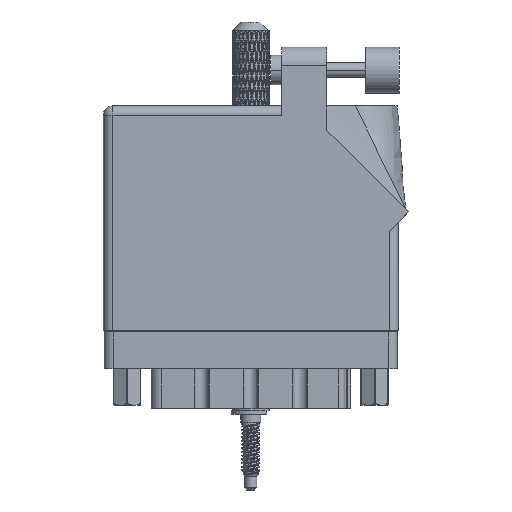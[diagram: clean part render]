
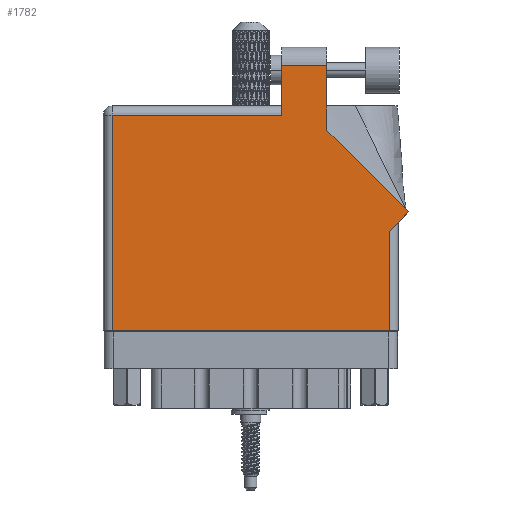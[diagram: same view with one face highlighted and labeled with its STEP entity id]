
A CAD part, front view. The second image highlights one B-rep face of the part: STEP entity #1782.
In plain terms, the highlighted face is planar.
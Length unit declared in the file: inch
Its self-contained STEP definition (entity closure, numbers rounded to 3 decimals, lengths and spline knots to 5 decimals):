
#1079 = CARTESIAN_POINT ( 'NONE',  ( 1.217, 1.468, 0. ) ) ;
#1595 = VERTEX_POINT ( 'NONE', #8621 ) ;
#1782 = ADVANCED_FACE ( 'NONE', ( #30222 ), #41674, .F. ) ;
#3000 = CARTESIAN_POINT ( 'NONE',  ( 1.524, 1.36442, 0. ) ) ;
#3484 = CARTESIAN_POINT ( 'NONE',  ( 0.062, 1.468, 0. ) ) ;
#4439 = DIRECTION ( 'NONE',  ( 0.707, 0.707, 0. ) ) ;
#5820 = DIRECTION ( 'NONE',  ( 0., 0., -1. ) ) ;
#7330 = CARTESIAN_POINT ( 'NONE',  ( 1.217, 1.805, 0. ) ) ;
#8535 = LINE ( 'NONE', #74243, #37819 ) ;
#8621 = CARTESIAN_POINT ( 'NONE',  ( 1.948, 0., 0. ) ) ;
#8852 = DIRECTION ( 'NONE',  ( -1., 0., 0. ) ) ;
#11209 = VERTEX_POINT ( 'NONE', #54632 ) ;
#14079 = CARTESIAN_POINT ( 'NONE',  ( 0., 0., 0. ) ) ;
#14585 = ORIENTED_EDGE ( 'NONE', *, *, #41358, .T. ) ;
#17971 = VECTOR ( 'NONE', #71233, 39.37008 ) ;
#21983 = EDGE_CURVE ( 'NONE', #82970, #11209, #63542, .T. ) ;
#24274 = VERTEX_POINT ( 'NONE', #65346 ) ;
#25549 = ORIENTED_EDGE ( 'NONE', *, *, #51403, .T. ) ;
#30222 = FACE_OUTER_BOUND ( 'NONE', #75222, .T. ) ;
#33409 = CARTESIAN_POINT ( 'NONE',  ( 1.217, 1.53, 0. ) ) ;
#34338 = VERTEX_POINT ( 'NONE', #101010 ) ;
#35198 = AXIS2_PLACEMENT_3D ( 'NONE', #96344, #5820, #78732 ) ;
#35311 = CARTESIAN_POINT ( 'NONE',  ( 1.948, 0.737, 0. ) ) ;
#35503 = EDGE_CURVE ( 'NONE', #1595, #34338, #65454, .T. ) ;
#37819 = VECTOR ( 'NONE', #55065, 39.37008 ) ;
#38905 = VERTEX_POINT ( 'NONE', #1079 ) ;
#39830 = VECTOR ( 'NONE', #8852, 39.37008 ) ;
#41358 = EDGE_CURVE ( 'NONE', #80848, #73430, #53424, .T. ) ;
#41674 = PLANE ( 'NONE',  #35198 ) ;
#43501 = ORIENTED_EDGE ( 'NONE', *, *, #80436, .T. ) ;
#51403 = EDGE_CURVE ( 'NONE', #11209, #38905, #78884, .T. ) ;
#52581 = DIRECTION ( 'NONE',  ( -1., 0., 0. ) ) ;
#53424 = LINE ( 'NONE', #67538, #74441 ) ;
#54254 = ORIENTED_EDGE ( 'NONE', *, *, #112278, .T. ) ;
#54556 = VECTOR ( 'NONE', #103477, 39.37008 ) ;
#54632 = CARTESIAN_POINT ( 'NONE',  ( 1.217, 1.805, 0. ) ) ;
#55065 = DIRECTION ( 'NONE',  ( 0., -1., 0. ) ) ;
#55110 = VECTOR ( 'NONE', #95131, 39.37008 ) ;
#57934 = ORIENTED_EDGE ( 'NONE', *, *, #21983, .T. ) ;
#59275 = CARTESIAN_POINT ( 'NONE',  ( 1.524, 1.36442, 0. ) ) ;
#61958 = VECTOR ( 'NONE', #52581, 39.37008 ) ;
#62720 = VECTOR ( 'NONE', #103461, 39.37008 ) ;
#63542 = LINE ( 'NONE', #7330, #39830 ) ;
#64389 = VERTEX_POINT ( 'NONE', #3484 ) ;
#65346 = CARTESIAN_POINT ( 'NONE',  ( 0.062, 0., 0. ) ) ;
#65454 = LINE ( 'NONE', #35311, #17971 ) ;
#65550 = LINE ( 'NONE', #59275, #62720 ) ;
#66986 = CARTESIAN_POINT ( 'NONE',  ( 1.524, 1.805, 0. ) ) ;
#67538 = CARTESIAN_POINT ( 'NONE',  ( 2.08071, 0.80771, 0. ) ) ;
#69007 = ORIENTED_EDGE ( 'NONE', *, *, #108070, .T. ) ;
#69476 = DIRECTION ( 'NONE',  ( -0.707, 0.707, 0. ) ) ;
#71139 = EDGE_CURVE ( 'NONE', #73430, #82970, #65550, .T. ) ;
#71233 = DIRECTION ( 'NONE',  ( 0., 1., 0. ) ) ;
#73430 = VERTEX_POINT ( 'NONE', #3000 ) ;
#74243 = CARTESIAN_POINT ( 'NONE',  ( 0.062, 0., 0. ) ) ;
#74441 = VECTOR ( 'NONE', #69476, 39.37008 ) ;
#75222 = EDGE_LOOP ( 'NONE', ( #113677, #57934, #25549, #69007, #43501, #96311, #83259, #54254, #14585 ) ) ;
#78732 = DIRECTION ( 'NONE',  ( -1., 0., 0. ) ) ;
#78884 = LINE ( 'NONE', #33409, #55110 ) ;
#80436 = EDGE_CURVE ( 'NONE', #64389, #24274, #8535, .T. ) ;
#80848 = VERTEX_POINT ( 'NONE', #96811 ) ;
#82970 = VERTEX_POINT ( 'NONE', #66986 ) ;
#83259 = ORIENTED_EDGE ( 'NONE', *, *, #35503, .T. ) ;
#84298 = LINE ( 'NONE', #114312, #61958 ) ;
#87863 = EDGE_CURVE ( 'NONE', #24274, #1595, #100769, .T. ) ;
#89475 = VECTOR ( 'NONE', #4439, 39.37008 ) ;
#94179 = CARTESIAN_POINT ( 'NONE',  ( 2.01, 0.737, 0. ) ) ;
#95131 = DIRECTION ( 'NONE',  ( 0., -1., 0. ) ) ;
#96311 = ORIENTED_EDGE ( 'NONE', *, *, #87863, .T. ) ;
#96344 = CARTESIAN_POINT ( 'NONE',  ( 0., 1.53, 0. ) ) ;
#96811 = CARTESIAN_POINT ( 'NONE',  ( 2.08071, 0.80771, 0. ) ) ;
#100769 = LINE ( 'NONE', #14079, #54556 ) ;
#101010 = CARTESIAN_POINT ( 'NONE',  ( 1.948, 0.675, 0. ) ) ;
#103461 = DIRECTION ( 'NONE',  ( 0., 1., 0. ) ) ;
#103477 = DIRECTION ( 'NONE',  ( 1., 0., 0. ) ) ;
#108070 = EDGE_CURVE ( 'NONE', #38905, #64389, #84298, .T. ) ;
#112278 = EDGE_CURVE ( 'NONE', #34338, #80848, #113267, .T. ) ;
#113267 = LINE ( 'NONE', #94179, #89475 ) ;
#113677 = ORIENTED_EDGE ( 'NONE', *, *, #71139, .T. ) ;
#114312 = CARTESIAN_POINT ( 'NONE',  ( 0., 1.468, 0. ) ) ;
